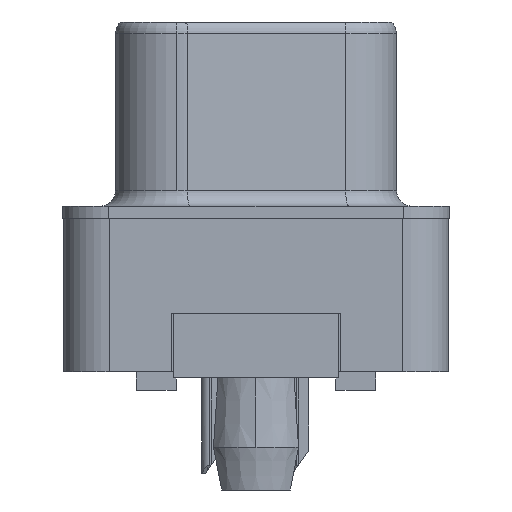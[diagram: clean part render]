
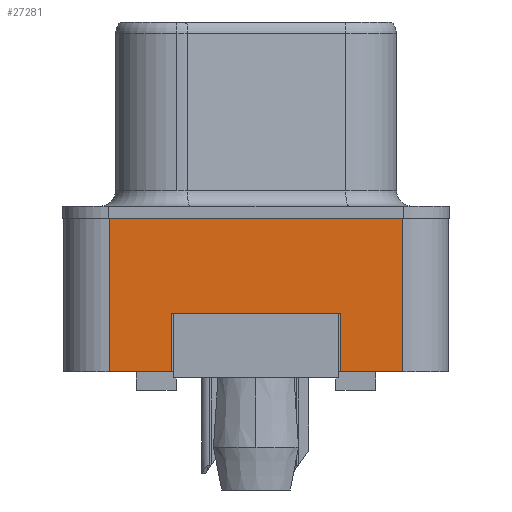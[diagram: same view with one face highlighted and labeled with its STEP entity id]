
A CAD part, left-side view. The second image highlights one B-rep face of the part: STEP entity #27281.
In plain terms, the highlighted planar face has unit normal (-1, 0, 0).
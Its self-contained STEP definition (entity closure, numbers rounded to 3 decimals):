
#581 = PLANE ( 'NONE',  #14334 ) ;
#619 = VERTEX_POINT ( 'NONE', #18432 ) ;
#1677 = DIRECTION ( 'NONE',  ( 0., 0., 1. ) ) ;
#2020 = VERTEX_POINT ( 'NONE', #17261 ) ;
#2308 = ORIENTED_EDGE ( 'NONE', *, *, #10722, .T. ) ;
#2322 = CARTESIAN_POINT ( 'NONE',  ( -2.91, -2.75, -3.1 ) ) ;
#2697 = CARTESIAN_POINT ( 'NONE',  ( -2.91, 2.75, -5. ) ) ;
#2899 = EDGE_CURVE ( 'NONE', #619, #2020, #21047, .T. ) ;
#2916 = EDGE_CURVE ( 'NONE', #25138, #619, #23854, .T. ) ;
#2957 = DIRECTION ( 'NONE',  ( 0., 0., 1. ) ) ;
#3572 = VERTEX_POINT ( 'NONE', #2322 ) ;
#3755 = CARTESIAN_POINT ( 'NONE',  ( -2.91, 2.75, -3.1 ) ) ;
#4462 = ORIENTED_EDGE ( 'NONE', *, *, #2916, .F. ) ;
#4708 = ORIENTED_EDGE ( 'NONE', *, *, #21425, .T. ) ;
#4979 = VERTEX_POINT ( 'NONE', #27190 ) ;
#5259 = LINE ( 'NONE', #28311, #27954 ) ;
#5347 = CARTESIAN_POINT ( 'NONE',  ( -2.91, 2.75, -3.1 ) ) ;
#5388 = VECTOR ( 'NONE', #24062, 1000. ) ;
#5394 = CARTESIAN_POINT ( 'NONE',  ( -2.91, 2.75, -3.1 ) ) ;
#6204 = EDGE_CURVE ( 'NONE', #14867, #22099, #10395, .T. ) ;
#7095 = CARTESIAN_POINT ( 'NONE',  ( -2.91, -4.775, -5. ) ) ;
#7994 = CARTESIAN_POINT ( 'NONE',  ( -2.91, 4.775, -5. ) ) ;
#8118 = EDGE_LOOP ( 'NONE', ( #19936, #4708, #2308, #14509, #4462, #22560, #25910, #11849 ) ) ;
#9671 = LINE ( 'NONE', #13529, #19175 ) ;
#9803 = DIRECTION ( 'NONE',  ( 0., -1., 0. ) ) ;
#9844 = VECTOR ( 'NONE', #9803, 1000. ) ;
#10048 = VERTEX_POINT ( 'NONE', #10071 ) ;
#10071 = CARTESIAN_POINT ( 'NONE',  ( -2.91, -4.775, -5. ) ) ;
#10395 = LINE ( 'NONE', #3755, #15253 ) ;
#10595 = VECTOR ( 'NONE', #14419, 1000. ) ;
#10722 = EDGE_CURVE ( 'NONE', #10048, #2020, #9671, .T. ) ;
#11725 = CARTESIAN_POINT ( 'NONE',  ( -2.91, -4.775, -5. ) ) ;
#11806 = FACE_OUTER_BOUND ( 'NONE', #8118, .T. ) ;
#11849 = ORIENTED_EDGE ( 'NONE', *, *, #28388, .F. ) ;
#12020 = LINE ( 'NONE', #11725, #23869 ) ;
#13298 = EDGE_CURVE ( 'NONE', #25138, #22099, #12020, .T. ) ;
#13529 = CARTESIAN_POINT ( 'NONE',  ( -2.91, -4.775, -5. ) ) ;
#14243 = CARTESIAN_POINT ( 'NONE',  ( -2.91, -4.775, 0. ) ) ;
#14334 = AXIS2_PLACEMENT_3D ( 'NONE', #7095, #27912, #2957 ) ;
#14419 = DIRECTION ( 'NONE',  ( 0., 1., 0. ) ) ;
#14509 = ORIENTED_EDGE ( 'NONE', *, *, #2899, .F. ) ;
#14867 = VERTEX_POINT ( 'NONE', #5347 ) ;
#15253 = VECTOR ( 'NONE', #17489, 1000. ) ;
#17261 = CARTESIAN_POINT ( 'NONE',  ( -2.91, -4.775, 0. ) ) ;
#17489 = DIRECTION ( 'NONE',  ( 0., 0., -1. ) ) ;
#17539 = CARTESIAN_POINT ( 'NONE',  ( -2.91, -2.75, -3.1 ) ) ;
#17878 = VECTOR ( 'NONE', #1677, 1000. ) ;
#18432 = CARTESIAN_POINT ( 'NONE',  ( -2.91, 4.775, 0. ) ) ;
#19175 = VECTOR ( 'NONE', #27120, 1000. ) ;
#19936 = ORIENTED_EDGE ( 'NONE', *, *, #24523, .T. ) ;
#21047 = LINE ( 'NONE', #14243, #9844 ) ;
#21227 = DIRECTION ( 'NONE',  ( 0., -1., 0. ) ) ;
#21342 = CARTESIAN_POINT ( 'NONE',  ( -2.91, 4.775, -5. ) ) ;
#21425 = EDGE_CURVE ( 'NONE', #4979, #10048, #5259, .T. ) ;
#22099 = VERTEX_POINT ( 'NONE', #2697 ) ;
#22560 = ORIENTED_EDGE ( 'NONE', *, *, #13298, .T. ) ;
#23427 = DIRECTION ( 'NONE',  ( 0., -1., 0. ) ) ;
#23854 = LINE ( 'NONE', #21342, #17878 ) ;
#23869 = VECTOR ( 'NONE', #23427, 1000. ) ;
#24062 = DIRECTION ( 'NONE',  ( 0., 0., -1. ) ) ;
#24523 = EDGE_CURVE ( 'NONE', #3572, #4979, #24623, .T. ) ;
#24623 = LINE ( 'NONE', #17539, #5388 ) ;
#25138 = VERTEX_POINT ( 'NONE', #7994 ) ;
#25636 = LINE ( 'NONE', #5394, #10595 ) ;
#25910 = ORIENTED_EDGE ( 'NONE', *, *, #6204, .F. ) ;
#27120 = DIRECTION ( 'NONE',  ( 0., 0., 1. ) ) ;
#27190 = CARTESIAN_POINT ( 'NONE',  ( -2.91, -2.75, -5. ) ) ;
#27281 = ADVANCED_FACE ( 'NONE', ( #11806 ), #581, .T. ) ;
#27912 = DIRECTION ( 'NONE',  ( -1., 0., 0. ) ) ;
#27954 = VECTOR ( 'NONE', #21227, 1000. ) ;
#28311 = CARTESIAN_POINT ( 'NONE',  ( -2.91, -4.775, -5. ) ) ;
#28388 = EDGE_CURVE ( 'NONE', #3572, #14867, #25636, .T. ) ;
